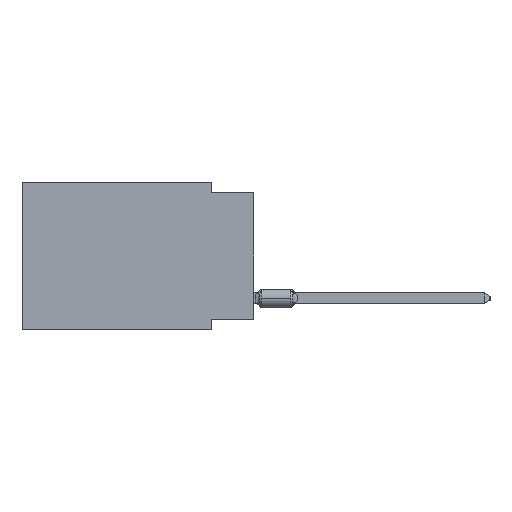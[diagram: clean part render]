
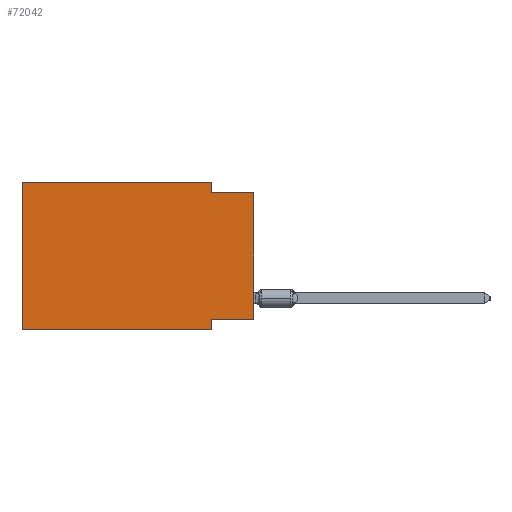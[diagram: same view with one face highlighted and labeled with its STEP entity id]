
A CAD part, left-side view. The second image highlights one B-rep face of the part: STEP entity #72042.
In plain terms, the highlighted planar face has unit normal (-1, 0, 0).
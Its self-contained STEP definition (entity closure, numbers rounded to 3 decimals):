
#632 = CARTESIAN_POINT ( 'NONE',  ( 0., 2.54, -8.89 ) ) ;
#917 = LINE ( 'NONE', #61646, #71181 ) ;
#1046 = LINE ( 'NONE', #29562, #16216 ) ;
#5219 = LINE ( 'NONE', #38860, #20240 ) ;
#5949 = ORIENTED_EDGE ( 'NONE', *, *, #53381, .F. ) ;
#6906 = DIRECTION ( 'NONE',  ( 0., 0., -1. ) ) ;
#7557 = ORIENTED_EDGE ( 'NONE', *, *, #67249, .F. ) ;
#7783 = VECTOR ( 'NONE', #41049, 1000. ) ;
#8720 = VERTEX_POINT ( 'NONE', #40462 ) ;
#10015 = CARTESIAN_POINT ( 'NONE',  ( 0., 13.97, 0. ) ) ;
#10296 = CARTESIAN_POINT ( 'NONE',  ( 0., 2.54, 0. ) ) ;
#12160 = LINE ( 'NONE', #45466, #7783 ) ;
#12914 = DIRECTION ( 'NONE',  ( 0., -1., 0. ) ) ;
#13279 = FACE_OUTER_BOUND ( 'NONE', #27170, .T. ) ;
#15100 = EDGE_CURVE ( 'NONE', #43032, #52098, #1046, .T. ) ;
#16216 = VECTOR ( 'NONE', #6906, 1000. ) ;
#17692 = DIRECTION ( 'NONE',  ( 0., 0., -1. ) ) ;
#20240 = VECTOR ( 'NONE', #34091, 1000. ) ;
#20797 = VERTEX_POINT ( 'NONE', #60280 ) ;
#21616 = VERTEX_POINT ( 'NONE', #632 ) ;
#24599 = CARTESIAN_POINT ( 'NONE',  ( 0., 13.97, 0. ) ) ;
#24898 = CARTESIAN_POINT ( 'NONE',  ( 0., 13.97, 0. ) ) ;
#25518 = EDGE_CURVE ( 'NONE', #52098, #8720, #12160, .T. ) ;
#26151 = VERTEX_POINT ( 'NONE', #37981 ) ;
#26834 = DIRECTION ( 'NONE',  ( 0., -1., 0. ) ) ;
#27170 = EDGE_LOOP ( 'NONE', ( #57465, #59742, #34283, #5949, #7557, #29508, #45151, #56371 ) ) ;
#29155 = EDGE_CURVE ( 'NONE', #20797, #21616, #53853, .T. ) ;
#29508 = ORIENTED_EDGE ( 'NONE', *, *, #42461, .T. ) ;
#29514 = CARTESIAN_POINT ( 'NONE',  ( 0., 0., -8.255 ) ) ;
#29562 = CARTESIAN_POINT ( 'NONE',  ( 0., 2.54, 0. ) ) ;
#30111 = PLANE ( 'NONE',  #67217 ) ;
#30689 = VERTEX_POINT ( 'NONE', #62659 ) ;
#31157 = DIRECTION ( 'NONE',  ( 0., 0., -1. ) ) ;
#34091 = DIRECTION ( 'NONE',  ( 0., 1., 0. ) ) ;
#34283 = ORIENTED_EDGE ( 'NONE', *, *, #15100, .F. ) ;
#34603 = EDGE_CURVE ( 'NONE', #36477, #8720, #917, .T. ) ;
#35950 = LINE ( 'NONE', #63045, #65563 ) ;
#36477 = VERTEX_POINT ( 'NONE', #29514 ) ;
#37981 = CARTESIAN_POINT ( 'NONE',  ( 0., 13.97, -8.89 ) ) ;
#38860 = CARTESIAN_POINT ( 'NONE',  ( 0., 0., -8.255 ) ) ;
#40462 = CARTESIAN_POINT ( 'NONE',  ( 0., 0., -0.635 ) ) ;
#41049 = DIRECTION ( 'NONE',  ( 0., -1., 0. ) ) ;
#42461 = EDGE_CURVE ( 'NONE', #26151, #21616, #35950, .T. ) ;
#42462 = LINE ( 'NONE', #24898, #67050 ) ;
#42680 = CARTESIAN_POINT ( 'NONE',  ( 0., 2.54, -0.635 ) ) ;
#43032 = VERTEX_POINT ( 'NONE', #10296 ) ;
#45151 = ORIENTED_EDGE ( 'NONE', *, *, #29155, .F. ) ;
#45466 = CARTESIAN_POINT ( 'NONE',  ( 0., 0., -0.635 ) ) ;
#46936 = DIRECTION ( 'NONE',  ( 1., 0., 0. ) ) ;
#47975 = DIRECTION ( 'NONE',  ( 0., 0., 1. ) ) ;
#52098 = VERTEX_POINT ( 'NONE', #42680 ) ;
#53381 = EDGE_CURVE ( 'NONE', #30689, #43032, #60142, .T. ) ;
#53853 = LINE ( 'NONE', #64095, #69593 ) ;
#54648 = VECTOR ( 'NONE', #26834, 1000. ) ;
#56371 = ORIENTED_EDGE ( 'NONE', *, *, #67039, .F. ) ;
#57465 = ORIENTED_EDGE ( 'NONE', *, *, #34603, .T. ) ;
#59742 = ORIENTED_EDGE ( 'NONE', *, *, #25518, .F. ) ;
#60142 = LINE ( 'NONE', #10015, #54648 ) ;
#60280 = CARTESIAN_POINT ( 'NONE',  ( 0., 2.54, -8.255 ) ) ;
#61282 = DIRECTION ( 'NONE',  ( 0., 0., 1. ) ) ;
#61646 = CARTESIAN_POINT ( 'NONE',  ( 0., 0., 0. ) ) ;
#62659 = CARTESIAN_POINT ( 'NONE',  ( 0., 13.97, 0. ) ) ;
#63045 = CARTESIAN_POINT ( 'NONE',  ( 0., 13.97, -8.89 ) ) ;
#64095 = CARTESIAN_POINT ( 'NONE',  ( 0., 2.54, -8.89 ) ) ;
#65563 = VECTOR ( 'NONE', #12914, 1000. ) ;
#67039 = EDGE_CURVE ( 'NONE', #36477, #20797, #5219, .T. ) ;
#67050 = VECTOR ( 'NONE', #47975, 1000. ) ;
#67217 = AXIS2_PLACEMENT_3D ( 'NONE', #24599, #46936, #17692 ) ;
#67249 = EDGE_CURVE ( 'NONE', #26151, #30689, #42462, .T. ) ;
#69593 = VECTOR ( 'NONE', #31157, 1000. ) ;
#71181 = VECTOR ( 'NONE', #61282, 1000. ) ;
#72042 = ADVANCED_FACE ( 'NONE', ( #13279 ), #30111, .F. ) ;
